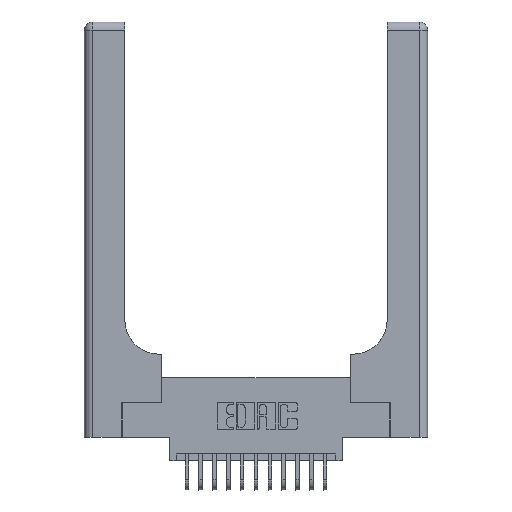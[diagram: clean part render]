
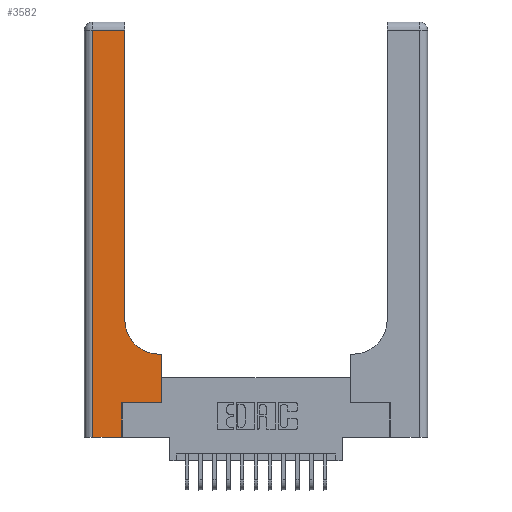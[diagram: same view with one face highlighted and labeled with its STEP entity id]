
A CAD part, top view. The second image highlights one B-rep face of the part: STEP entity #3582.
In plain terms, the highlighted planar face has unit normal (0, 0, 1).
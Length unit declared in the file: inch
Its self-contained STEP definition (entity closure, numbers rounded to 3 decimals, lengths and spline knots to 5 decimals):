
#427 = CARTESIAN_POINT ( 'NONE',  ( 0.269, 0., 0.37 ) ) ;
#483 = EDGE_CURVE ( 'NONE', #7418, #772, #10829, .T. ) ;
#750 = EDGE_CURVE ( 'NONE', #14774, #2627, #11299, .T. ) ;
#772 = VERTEX_POINT ( 'NONE', #17229 ) ;
#1187 = CARTESIAN_POINT ( 'NONE',  ( 0.269, 0.25, 0.37 ) ) ;
#1539 = CARTESIAN_POINT ( 'NONE',  ( 0.5415, 0.85, 0.37 ) ) ;
#1565 = ORIENTED_EDGE ( 'NONE', *, *, #2205, .T. ) ;
#2205 = EDGE_CURVE ( 'NONE', #4405, #11845, #3568, .T. ) ;
#2516 = CARTESIAN_POINT ( 'NONE',  ( 0.2915, 0.6, 0.37 ) ) ;
#2627 = VERTEX_POINT ( 'NONE', #19212 ) ;
#2957 = LINE ( 'NONE', #8793, #17033 ) ;
#3120 = DIRECTION ( 'NONE',  ( 1., 0., 0. ) ) ;
#3568 = CIRCLE ( 'NONE', #11678, 0.25 ) ;
#3582 = ADVANCED_FACE ( 'NONE', ( #7323 ), #9552, .F. ) ;
#3725 = LINE ( 'NONE', #18139, #9973 ) ;
#4405 = VERTEX_POINT ( 'NONE', #5516 ) ;
#4559 = VECTOR ( 'NONE', #19263, 39.37008 ) ;
#4599 = VERTEX_POINT ( 'NONE', #15866 ) ;
#4651 = EDGE_CURVE ( 'NONE', #2627, #7418, #8983, .T. ) ;
#4735 = ORIENTED_EDGE ( 'NONE', *, *, #8061, .T. ) ;
#5013 = AXIS2_PLACEMENT_3D ( 'NONE', #17506, #9963, #8397 ) ;
#5516 = CARTESIAN_POINT ( 'NONE',  ( 0.5415, 0.6, 0.37 ) ) ;
#5681 = VERTEX_POINT ( 'NONE', #8238 ) ;
#7207 = VECTOR ( 'NONE', #14058, 39.37008 ) ;
#7323 = FACE_OUTER_BOUND ( 'NONE', #16447, .T. ) ;
#7418 = VERTEX_POINT ( 'NONE', #427 ) ;
#8061 = EDGE_CURVE ( 'NONE', #4599, #4405, #18864, .T. ) ;
#8238 = CARTESIAN_POINT ( 'NONE',  ( 0.2915, 2.94, 0.37 ) ) ;
#8254 = VECTOR ( 'NONE', #8470, 39.37008 ) ;
#8397 = DIRECTION ( 'NONE',  ( -1., 0., 0. ) ) ;
#8470 = DIRECTION ( 'NONE',  ( 1., 0., 0. ) ) ;
#8793 = CARTESIAN_POINT ( 'NONE',  ( 0., 2.94, 0.37 ) ) ;
#8983 = LINE ( 'NONE', #11285, #8254 ) ;
#9038 = DIRECTION ( 'NONE',  ( 0., 1., 0. ) ) ;
#9098 = DIRECTION ( 'NONE',  ( 0., 1., 0. ) ) ;
#9152 = VECTOR ( 'NONE', #9098, 39.37008 ) ;
#9552 = PLANE ( 'NONE',  #5013 ) ;
#9963 = DIRECTION ( 'NONE',  ( 0., 0., -1. ) ) ;
#9973 = VECTOR ( 'NONE', #15239, 39.37008 ) ;
#10829 = LINE ( 'NONE', #12088, #9152 ) ;
#11038 = EDGE_CURVE ( 'NONE', #772, #15740, #12326, .T. ) ;
#11234 = CARTESIAN_POINT ( 'NONE',  ( 0.06, 2.94, 0.37 ) ) ;
#11285 = CARTESIAN_POINT ( 'NONE',  ( 0., 0., 0.37 ) ) ;
#11299 = LINE ( 'NONE', #18835, #7207 ) ;
#11678 = AXIS2_PLACEMENT_3D ( 'NONE', #1539, #12299, #3120 ) ;
#11814 = DIRECTION ( 'NONE',  ( 1., 0., 0. ) ) ;
#11844 = ORIENTED_EDGE ( 'NONE', *, *, #15709, .T. ) ;
#11845 = VERTEX_POINT ( 'NONE', #18627 ) ;
#11902 = ORIENTED_EDGE ( 'NONE', *, *, #11038, .T. ) ;
#12088 = CARTESIAN_POINT ( 'NONE',  ( 0.269, 0., 0.37 ) ) ;
#12299 = DIRECTION ( 'NONE',  ( 0., 0., -1. ) ) ;
#12326 = LINE ( 'NONE', #1187, #13506 ) ;
#13362 = ORIENTED_EDGE ( 'NONE', *, *, #483, .T. ) ;
#13506 = VECTOR ( 'NONE', #11814, 39.37008 ) ;
#13664 = VECTOR ( 'NONE', #9038, 39.37008 ) ;
#13897 = EDGE_CURVE ( 'NONE', #11845, #5681, #3725, .T. ) ;
#14058 = DIRECTION ( 'NONE',  ( 0., -1., 0. ) ) ;
#14774 = VERTEX_POINT ( 'NONE', #11234 ) ;
#14864 = DIRECTION ( 'NONE',  ( -1., 0., 0. ) ) ;
#15021 = CARTESIAN_POINT ( 'NONE',  ( 0.5585, 0.25, 0.37 ) ) ;
#15239 = DIRECTION ( 'NONE',  ( 0., 1., 0. ) ) ;
#15709 = EDGE_CURVE ( 'NONE', #5681, #14774, #2957, .T. ) ;
#15740 = VERTEX_POINT ( 'NONE', #19323 ) ;
#15866 = CARTESIAN_POINT ( 'NONE',  ( 0.5585, 0.6, 0.37 ) ) ;
#15874 = ORIENTED_EDGE ( 'NONE', *, *, #4651, .T. ) ;
#16447 = EDGE_LOOP ( 'NONE', ( #16993, #11844, #19398, #15874, #13362, #11902, #19791, #4735, #1565 ) ) ;
#16787 = EDGE_CURVE ( 'NONE', #15740, #4599, #19644, .T. ) ;
#16993 = ORIENTED_EDGE ( 'NONE', *, *, #13897, .T. ) ;
#17033 = VECTOR ( 'NONE', #14864, 39.37008 ) ;
#17229 = CARTESIAN_POINT ( 'NONE',  ( 0.269, 0.25, 0.37 ) ) ;
#17506 = CARTESIAN_POINT ( 'NONE',  ( 0., 3., 0.37 ) ) ;
#18139 = CARTESIAN_POINT ( 'NONE',  ( 0.2915, 3., 0.37 ) ) ;
#18627 = CARTESIAN_POINT ( 'NONE',  ( 0.2915, 0.85, 0.37 ) ) ;
#18835 = CARTESIAN_POINT ( 'NONE',  ( 0.06, 3., 0.37 ) ) ;
#18864 = LINE ( 'NONE', #2516, #4559 ) ;
#19212 = CARTESIAN_POINT ( 'NONE',  ( 0.06, 0., 0.37 ) ) ;
#19263 = DIRECTION ( 'NONE',  ( -1., 0., 0. ) ) ;
#19323 = CARTESIAN_POINT ( 'NONE',  ( 0.5585, 0.25, 0.37 ) ) ;
#19398 = ORIENTED_EDGE ( 'NONE', *, *, #750, .T. ) ;
#19644 = LINE ( 'NONE', #15021, #13664 ) ;
#19791 = ORIENTED_EDGE ( 'NONE', *, *, #16787, .T. ) ;
